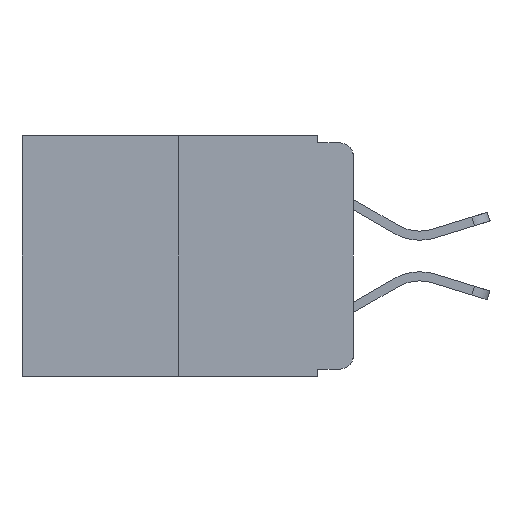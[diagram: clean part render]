
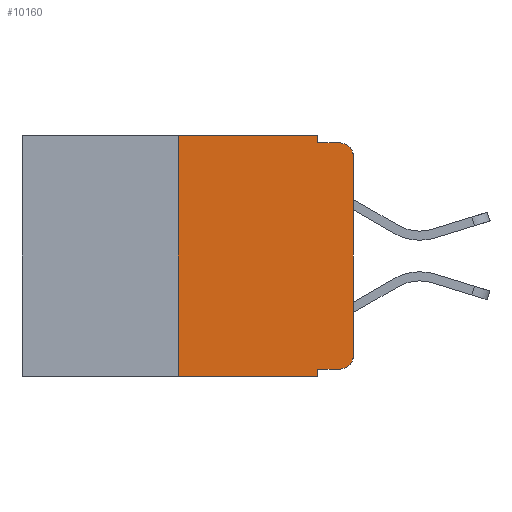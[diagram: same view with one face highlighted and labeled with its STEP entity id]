
A CAD part, left-side view. The second image highlights one B-rep face of the part: STEP entity #10160.
In plain terms, the highlighted planar face has unit normal (-1, 0, 0).
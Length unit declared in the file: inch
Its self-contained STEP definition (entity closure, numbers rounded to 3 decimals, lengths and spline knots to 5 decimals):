
#17 = CIRCLE ( 'NONE', #7253, 0.02 ) ;
#372 = DIRECTION ( 'NONE',  ( 0., 0., -1. ) ) ;
#724 = LINE ( 'NONE', #13778, #15994 ) ;
#837 = LINE ( 'NONE', #8059, #8462 ) ;
#942 = ORIENTED_EDGE ( 'NONE', *, *, #13913, .F. ) ;
#1171 = CARTESIAN_POINT ( 'NONE',  ( 0., 0.25, 0. ) ) ;
#1234 = PLANE ( 'NONE',  #6836 ) ;
#1252 = CARTESIAN_POINT ( 'NONE',  ( 0., 0.02, -0.03 ) ) ;
#1410 = DIRECTION ( 'NONE',  ( 0., 0., -1. ) ) ;
#1476 = VERTEX_POINT ( 'NONE', #17122 ) ;
#1576 = CARTESIAN_POINT ( 'NONE',  ( 0., 0.02, -0.333 ) ) ;
#1670 = EDGE_CURVE ( 'NONE', #13379, #3101, #18759, .T. ) ;
#2402 = ORIENTED_EDGE ( 'NONE', *, *, #3767, .T. ) ;
#2461 = CARTESIAN_POINT ( 'NONE',  ( 0., 0.473, 0. ) ) ;
#2598 = LINE ( 'NONE', #15736, #14365 ) ;
#2636 = DIRECTION ( 'NONE',  ( -1., 0., 0. ) ) ;
#3010 = CARTESIAN_POINT ( 'NONE',  ( 0., 0.051, -0.343 ) ) ;
#3099 = VERTEX_POINT ( 'NONE', #5610 ) ;
#3101 = VERTEX_POINT ( 'NONE', #7937 ) ;
#3636 = ORIENTED_EDGE ( 'NONE', *, *, #9392, .F. ) ;
#3682 = VERTEX_POINT ( 'NONE', #17451 ) ;
#3767 = EDGE_CURVE ( 'NONE', #3101, #8706, #12713, .T. ) ;
#4028 = EDGE_CURVE ( 'NONE', #17728, #13379, #17, .T. ) ;
#4600 = ORIENTED_EDGE ( 'NONE', *, *, #12277, .F. ) ;
#4778 = CARTESIAN_POINT ( 'NONE',  ( 0., 0.051, -0.01 ) ) ;
#4812 = CARTESIAN_POINT ( 'NONE',  ( 0., 0.051, -0.333 ) ) ;
#4858 = LINE ( 'NONE', #4812, #8809 ) ;
#5045 = DIRECTION ( 'NONE',  ( 0., 0., 1. ) ) ;
#5080 = VECTOR ( 'NONE', #5139, 39.37008 ) ;
#5139 = DIRECTION ( 'NONE',  ( 0., -1., 0. ) ) ;
#5610 = CARTESIAN_POINT ( 'NONE',  ( 0., 0.051, 0. ) ) ;
#6639 = CARTESIAN_POINT ( 'NONE',  ( 0., 0.25, 0. ) ) ;
#6836 = AXIS2_PLACEMENT_3D ( 'NONE', #8797, #7310, #11705 ) ;
#6946 = ORIENTED_EDGE ( 'NONE', *, *, #13236, .F. ) ;
#7052 = DIRECTION ( 'NONE',  ( 0., -1., 0. ) ) ;
#7106 = DIRECTION ( 'NONE',  ( 0., -1., 0. ) ) ;
#7253 = AXIS2_PLACEMENT_3D ( 'NONE', #18918, #10419, #1410 ) ;
#7310 = DIRECTION ( 'NONE',  ( 1., 0., 0. ) ) ;
#7766 = DIRECTION ( 'NONE',  ( 0., 0., 1. ) ) ;
#7924 = EDGE_CURVE ( 'NONE', #1476, #12057, #9489, .T. ) ;
#7937 = CARTESIAN_POINT ( 'NONE',  ( 0., 0., -0.03 ) ) ;
#8059 = CARTESIAN_POINT ( 'NONE',  ( 0., 0.051, 0. ) ) ;
#8405 = VERTEX_POINT ( 'NONE', #4778 ) ;
#8416 = CARTESIAN_POINT ( 'NONE',  ( 0., 0., -0.313 ) ) ;
#8462 = VECTOR ( 'NONE', #18076, 39.37008 ) ;
#8706 = VERTEX_POINT ( 'NONE', #17104 ) ;
#8797 = CARTESIAN_POINT ( 'NONE',  ( 0., 0.473, 0. ) ) ;
#8809 = VECTOR ( 'NONE', #14989, 39.37008 ) ;
#9392 = EDGE_CURVE ( 'NONE', #8405, #8706, #2598, .T. ) ;
#9489 = LINE ( 'NONE', #12488, #5080 ) ;
#9927 = VECTOR ( 'NONE', #7052, 39.37008 ) ;
#10160 = ADVANCED_FACE ( 'NONE', ( #11868 ), #1234, .F. ) ;
#10373 = VECTOR ( 'NONE', #5045, 39.37008 ) ;
#10419 = DIRECTION ( 'NONE',  ( -1., 0., 0. ) ) ;
#10550 = AXIS2_PLACEMENT_3D ( 'NONE', #1252, #2636, #372 ) ;
#10610 = ORIENTED_EDGE ( 'NONE', *, *, #7924, .T. ) ;
#11673 = VECTOR ( 'NONE', #7766, 39.37008 ) ;
#11705 = DIRECTION ( 'NONE',  ( 0., 0., -1. ) ) ;
#11868 = FACE_OUTER_BOUND ( 'NONE', #16218, .T. ) ;
#11948 = VERTEX_POINT ( 'NONE', #1171 ) ;
#12057 = VERTEX_POINT ( 'NONE', #3010 ) ;
#12277 = EDGE_CURVE ( 'NONE', #3099, #8405, #724, .T. ) ;
#12488 = CARTESIAN_POINT ( 'NONE',  ( 0., 0.473, -0.343 ) ) ;
#12713 = CIRCLE ( 'NONE', #10550, 0.02 ) ;
#13124 = CARTESIAN_POINT ( 'NONE',  ( 0., 0., 0. ) ) ;
#13236 = EDGE_CURVE ( 'NONE', #1476, #11948, #17479, .T. ) ;
#13379 = VERTEX_POINT ( 'NONE', #8416 ) ;
#13778 = CARTESIAN_POINT ( 'NONE',  ( 0., 0.051, 0. ) ) ;
#13913 = EDGE_CURVE ( 'NONE', #11948, #3099, #17483, .T. ) ;
#14365 = VECTOR ( 'NONE', #7106, 39.37008 ) ;
#14989 = DIRECTION ( 'NONE',  ( 0., -1., 0. ) ) ;
#15251 = DIRECTION ( 'NONE',  ( 0., 0., -1. ) ) ;
#15273 = ORIENTED_EDGE ( 'NONE', *, *, #1670, .T. ) ;
#15736 = CARTESIAN_POINT ( 'NONE',  ( 0., 0.051, -0.01 ) ) ;
#15994 = VECTOR ( 'NONE', #15251, 39.37008 ) ;
#16088 = EDGE_CURVE ( 'NONE', #3682, #12057, #837, .T. ) ;
#16218 = EDGE_LOOP ( 'NONE', ( #15273, #2402, #3636, #4600, #942, #6946, #10610, #18611, #16630, #17074 ) ) ;
#16630 = ORIENTED_EDGE ( 'NONE', *, *, #18922, .T. ) ;
#17074 = ORIENTED_EDGE ( 'NONE', *, *, #4028, .T. ) ;
#17104 = CARTESIAN_POINT ( 'NONE',  ( 0., 0.02, -0.01 ) ) ;
#17122 = CARTESIAN_POINT ( 'NONE',  ( 0., 0.25, -0.343 ) ) ;
#17451 = CARTESIAN_POINT ( 'NONE',  ( 0., 0.051, -0.333 ) ) ;
#17479 = LINE ( 'NONE', #6639, #10373 ) ;
#17483 = LINE ( 'NONE', #2461, #9927 ) ;
#17728 = VERTEX_POINT ( 'NONE', #1576 ) ;
#18076 = DIRECTION ( 'NONE',  ( 0., 0., -1. ) ) ;
#18611 = ORIENTED_EDGE ( 'NONE', *, *, #16088, .F. ) ;
#18759 = LINE ( 'NONE', #13124, #11673 ) ;
#18918 = CARTESIAN_POINT ( 'NONE',  ( 0., 0.02, -0.313 ) ) ;
#18922 = EDGE_CURVE ( 'NONE', #3682, #17728, #4858, .T. ) ;
